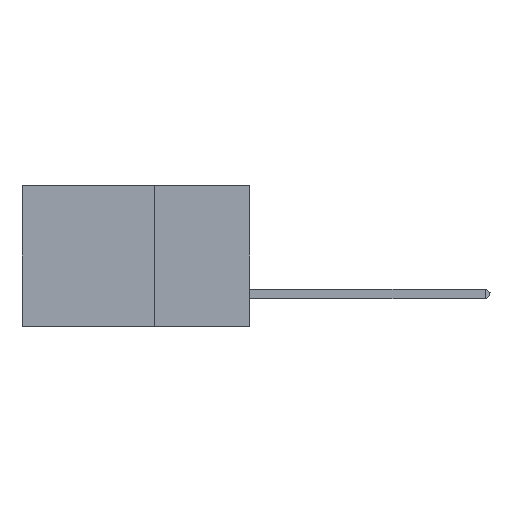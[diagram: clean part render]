
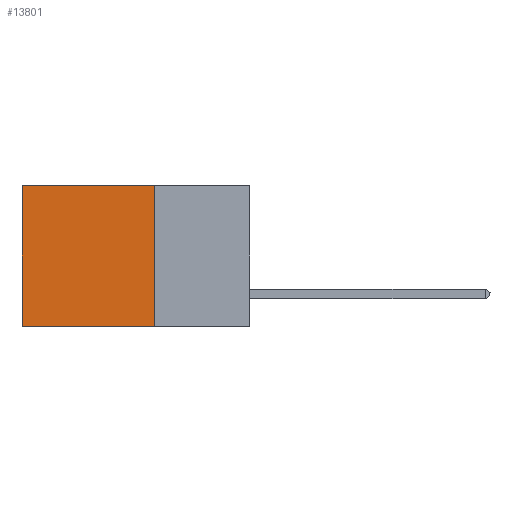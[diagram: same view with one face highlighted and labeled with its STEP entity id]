
A CAD part, left-side view. The second image highlights one B-rep face of the part: STEP entity #13801.
In plain terms, the highlighted planar face has unit normal (-1, 0, 0).
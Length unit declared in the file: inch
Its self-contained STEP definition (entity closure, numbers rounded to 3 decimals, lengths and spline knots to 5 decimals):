
#455 = VECTOR ( 'NONE', #6170, 39.37008 ) ;
#882 = LINE ( 'NONE', #1134, #455 ) ;
#1134 = CARTESIAN_POINT ( 'NONE',  ( 0.2875, 0.25, 0. ) ) ;
#2700 = CARTESIAN_POINT ( 'NONE',  ( 0.2875, 0.25, 0. ) ) ;
#3497 = ORIENTED_EDGE ( 'NONE', *, *, #13524, .F. ) ;
#3935 = FACE_OUTER_BOUND ( 'NONE', #5612, .T. ) ;
#4172 = PLANE ( 'NONE',  #7513 ) ;
#5390 = EDGE_CURVE ( 'NONE', #15842, #10892, #6938, .T. ) ;
#5612 = EDGE_LOOP ( 'NONE', ( #9934, #3497, #7776, #12808 ) ) ;
#6170 = DIRECTION ( 'NONE',  ( 0., 1., 0. ) ) ;
#6172 = CARTESIAN_POINT ( 'NONE',  ( 0.2875, 0.25, 0. ) ) ;
#6532 = VECTOR ( 'NONE', #11869, 39.37008 ) ;
#6704 = CARTESIAN_POINT ( 'NONE',  ( 0.2875, 0.6, 0. ) ) ;
#6938 = LINE ( 'NONE', #6704, #6532 ) ;
#7197 = CARTESIAN_POINT ( 'NONE',  ( 0.2875, 0.25, 0. ) ) ;
#7513 = AXIS2_PLACEMENT_3D ( 'NONE', #2700, #8873, #11603 ) ;
#7776 = ORIENTED_EDGE ( 'NONE', *, *, #15310, .F. ) ;
#8431 = VECTOR ( 'NONE', #9696, 39.37008 ) ;
#8539 = CARTESIAN_POINT ( 'NONE',  ( 0.2875, 0.6, 0. ) ) ;
#8873 = DIRECTION ( 'NONE',  ( 1., 0., 0. ) ) ;
#9142 = LINE ( 'NONE', #14060, #10101 ) ;
#9696 = DIRECTION ( 'NONE',  ( 0., 0., -1. ) ) ;
#9934 = ORIENTED_EDGE ( 'NONE', *, *, #5390, .T. ) ;
#10101 = VECTOR ( 'NONE', #15816, 39.37008 ) ;
#10892 = VERTEX_POINT ( 'NONE', #14195 ) ;
#11550 = EDGE_CURVE ( 'NONE', #12803, #15842, #882, .T. ) ;
#11603 = DIRECTION ( 'NONE',  ( 0., 0., -1. ) ) ;
#11869 = DIRECTION ( 'NONE',  ( 0., 0., -1. ) ) ;
#12028 = CARTESIAN_POINT ( 'NONE',  ( 0.2875, 0.25, -0.37 ) ) ;
#12803 = VERTEX_POINT ( 'NONE', #6172 ) ;
#12808 = ORIENTED_EDGE ( 'NONE', *, *, #11550, .T. ) ;
#13524 = EDGE_CURVE ( 'NONE', #13563, #10892, #9142, .T. ) ;
#13563 = VERTEX_POINT ( 'NONE', #12028 ) ;
#13801 = ADVANCED_FACE ( 'NONE', ( #3935 ), #4172, .F. ) ;
#14060 = CARTESIAN_POINT ( 'NONE',  ( 0.2875, 0.25, -0.37 ) ) ;
#14195 = CARTESIAN_POINT ( 'NONE',  ( 0.2875, 0.6, -0.37 ) ) ;
#14548 = LINE ( 'NONE', #7197, #8431 ) ;
#15310 = EDGE_CURVE ( 'NONE', #12803, #13563, #14548, .T. ) ;
#15816 = DIRECTION ( 'NONE',  ( 0., 1., 0. ) ) ;
#15842 = VERTEX_POINT ( 'NONE', #8539 ) ;
